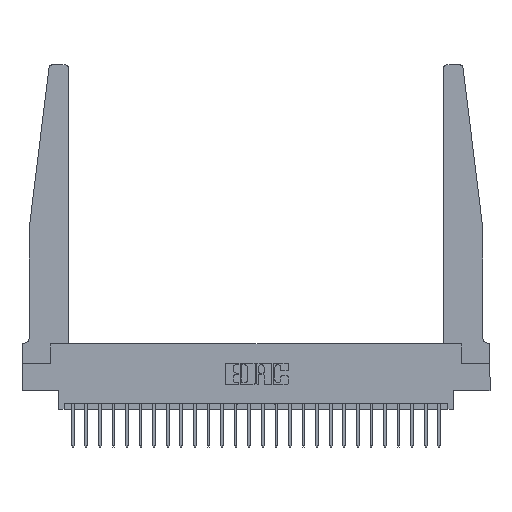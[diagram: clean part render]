
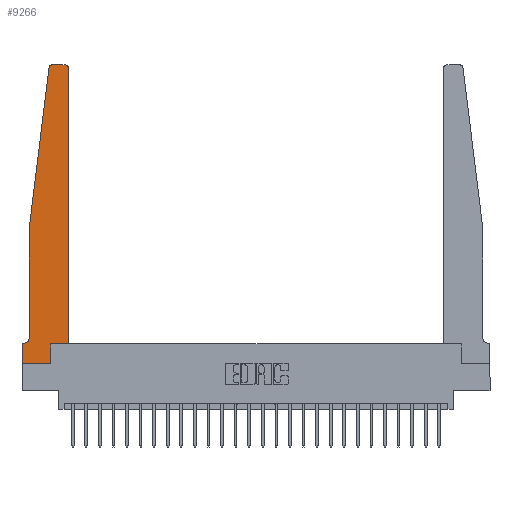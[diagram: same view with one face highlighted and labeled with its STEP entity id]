
A CAD part, top view. The second image highlights one B-rep face of the part: STEP entity #9266.
In plain terms, the highlighted planar face has unit normal (0, 0, 1).
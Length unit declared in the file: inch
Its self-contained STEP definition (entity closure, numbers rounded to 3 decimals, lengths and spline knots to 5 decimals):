
#272 = ORIENTED_EDGE ( 'NONE', *, *, #14787, .T. ) ;
#469 = EDGE_CURVE ( 'NONE', #1598, #17862, #11329, .T. ) ;
#521 = DIRECTION ( 'NONE',  ( -0.122, -0.992, 0. ) ) ;
#1453 = EDGE_CURVE ( 'NONE', #22445, #1598, #14292, .T. ) ;
#1598 = VERTEX_POINT ( 'NONE', #15333 ) ;
#2372 = CARTESIAN_POINT ( 'NONE',  ( 0.065, 0.1875, 0.37 ) ) ;
#2399 = EDGE_CURVE ( 'NONE', #22223, #10995, #5107, .T. ) ;
#2523 = EDGE_CURVE ( 'NONE', #14954, #24318, #22716, .T. ) ;
#2830 = CARTESIAN_POINT ( 'NONE',  ( 0., 0.1875, 0.37 ) ) ;
#2934 = EDGE_CURVE ( 'NONE', #22909, #4610, #3886, .T. ) ;
#3009 = CARTESIAN_POINT ( 'NONE',  ( 0.24675, 2.72367, 0.37 ) ) ;
#3243 = DIRECTION ( 'NONE',  ( 1., 0., 0. ) ) ;
#3268 = CARTESIAN_POINT ( 'NONE',  ( 0.2605, 0.18, 0.37 ) ) ;
#3551 = LINE ( 'NONE', #21809, #23583 ) ;
#3886 = LINE ( 'NONE', #2372, #8434 ) ;
#4200 = ORIENTED_EDGE ( 'NONE', *, *, #2934, .T. ) ;
#4582 = AXIS2_PLACEMENT_3D ( 'NONE', #4641, #18263, #6617 ) ;
#4610 = VERTEX_POINT ( 'NONE', #12937 ) ;
#4641 = CARTESIAN_POINT ( 'NONE',  ( 0.395, 2.72, 0.37 ) ) ;
#4689 = CARTESIAN_POINT ( 'NONE',  ( 0.425, 0.18, 0.37 ) ) ;
#4763 = ORIENTED_EDGE ( 'NONE', *, *, #2399, .T. ) ;
#4767 = EDGE_CURVE ( 'NONE', #17862, #22223, #10786, .T. ) ;
#4789 = ORIENTED_EDGE ( 'NONE', *, *, #11882, .T. ) ;
#4875 = CIRCLE ( 'NONE', #15342, 0.05 ) ;
#5107 = CIRCLE ( 'NONE', #4582, 0.03 ) ;
#5318 = CARTESIAN_POINT ( 'NONE',  ( 0.425, 0.18, 0.37 ) ) ;
#6133 = VECTOR ( 'NONE', #21604, 39.37008 ) ;
#6617 = DIRECTION ( 'NONE',  ( 1., 0., 0. ) ) ;
#6689 = EDGE_CURVE ( 'NONE', #12760, #16918, #17089, .T. ) ;
#6727 = DIRECTION ( 'NONE',  ( 1., 0., 0. ) ) ;
#6923 = CARTESIAN_POINT ( 'NONE',  ( 0.2605, 0., 0.37 ) ) ;
#7419 = CARTESIAN_POINT ( 'NONE',  ( 0.395, 2.75, 0.37 ) ) ;
#8035 = CARTESIAN_POINT ( 'NONE',  ( 0., 0., 0.37 ) ) ;
#8206 = DIRECTION ( 'NONE',  ( -1., 0., 0. ) ) ;
#8298 = CARTESIAN_POINT ( 'NONE',  ( 0.015, 0.2375, 0.37 ) ) ;
#8434 = VECTOR ( 'NONE', #8206, 39.37008 ) ;
#8600 = PLANE ( 'NONE',  #14808 ) ;
#8695 = CARTESIAN_POINT ( 'NONE',  ( 0.25, 2.75, 0.37 ) ) ;
#9102 = VECTOR ( 'NONE', #20760, 39.37008 ) ;
#9266 = ADVANCED_FACE ( 'NONE', ( #24094 ), #8600, .T. ) ;
#9939 = VECTOR ( 'NONE', #3243, 39.37008 ) ;
#10275 = DIRECTION ( 'NONE',  ( -1., 0., 0. ) ) ;
#10508 = EDGE_LOOP ( 'NONE', ( #20583, #14838, #272, #15156, #4789, #4200, #24207, #13949, #18498, #13337, #10584, #4763 ) ) ;
#10542 = EDGE_CURVE ( 'NONE', #4610, #22174, #12548, .T. ) ;
#10584 = ORIENTED_EDGE ( 'NONE', *, *, #4767, .T. ) ;
#10786 = LINE ( 'NONE', #5318, #20489 ) ;
#10872 = CARTESIAN_POINT ( 'NONE',  ( 0.27653, 2.72, 0.37 ) ) ;
#10995 = VERTEX_POINT ( 'NONE', #7419 ) ;
#11329 = LINE ( 'NONE', #13200, #17106 ) ;
#11882 = EDGE_CURVE ( 'NONE', #16918, #22909, #4875, .T. ) ;
#11920 = VECTOR ( 'NONE', #18100, 39.37008 ) ;
#12227 = CARTESIAN_POINT ( 'NONE',  ( 0.425, 2.72, 0.37 ) ) ;
#12236 = CARTESIAN_POINT ( 'NONE',  ( 0.065, 1.25, 0.37 ) ) ;
#12548 = LINE ( 'NONE', #8035, #6133 ) ;
#12760 = VERTEX_POINT ( 'NONE', #24766 ) ;
#12839 = DIRECTION ( 'NONE',  ( 1., 0., 0. ) ) ;
#12868 = CARTESIAN_POINT ( 'NONE',  ( 0., 0., 0.37 ) ) ;
#12937 = CARTESIAN_POINT ( 'NONE',  ( 0., 0.1875, 0.37 ) ) ;
#13200 = CARTESIAN_POINT ( 'NONE',  ( 0.425, 0.18, 0.37 ) ) ;
#13284 = DIRECTION ( 'NONE',  ( 1., 0., 0. ) ) ;
#13337 = ORIENTED_EDGE ( 'NONE', *, *, #469, .T. ) ;
#13538 = LINE ( 'NONE', #8695, #23221 ) ;
#13888 = CARTESIAN_POINT ( 'NONE',  ( 0.015, 0.1875, 0.37 ) ) ;
#13949 = ORIENTED_EDGE ( 'NONE', *, *, #24907, .T. ) ;
#14292 = LINE ( 'NONE', #3268, #9102 ) ;
#14787 = EDGE_CURVE ( 'NONE', #24318, #12760, #3551, .T. ) ;
#14808 = AXIS2_PLACEMENT_3D ( 'NONE', #2830, #18379, #6727 ) ;
#14838 = ORIENTED_EDGE ( 'NONE', *, *, #2523, .T. ) ;
#14954 = VERTEX_POINT ( 'NONE', #18417 ) ;
#15093 = LINE ( 'NONE', #12868, #9939 ) ;
#15156 = ORIENTED_EDGE ( 'NONE', *, *, #6689, .T. ) ;
#15333 = CARTESIAN_POINT ( 'NONE',  ( 0.2605, 0.18, 0.37 ) ) ;
#15342 = AXIS2_PLACEMENT_3D ( 'NONE', #8298, #21885, #10275 ) ;
#15537 = EDGE_CURVE ( 'NONE', #10995, #14954, #13538, .T. ) ;
#16356 = AXIS2_PLACEMENT_3D ( 'NONE', #10872, #24392, #12839 ) ;
#16918 = VERTEX_POINT ( 'NONE', #17685 ) ;
#17089 = LINE ( 'NONE', #12236, #11920 ) ;
#17106 = VECTOR ( 'NONE', #13284, 39.37008 ) ;
#17685 = CARTESIAN_POINT ( 'NONE',  ( 0.065, 0.2375, 0.37 ) ) ;
#17862 = VERTEX_POINT ( 'NONE', #4689 ) ;
#17925 = CARTESIAN_POINT ( 'NONE',  ( 0., 0., 0.37 ) ) ;
#18100 = DIRECTION ( 'NONE',  ( 0., -1., 0. ) ) ;
#18263 = DIRECTION ( 'NONE',  ( 0., 0., 1. ) ) ;
#18379 = DIRECTION ( 'NONE',  ( 0., 0., 1. ) ) ;
#18417 = CARTESIAN_POINT ( 'NONE',  ( 0.27653, 2.75, 0.37 ) ) ;
#18498 = ORIENTED_EDGE ( 'NONE', *, *, #1453, .T. ) ;
#20331 = DIRECTION ( 'NONE',  ( -1., 0., 0. ) ) ;
#20489 = VECTOR ( 'NONE', #23236, 39.37008 ) ;
#20583 = ORIENTED_EDGE ( 'NONE', *, *, #15537, .T. ) ;
#20760 = DIRECTION ( 'NONE',  ( 0., 1., 0. ) ) ;
#21604 = DIRECTION ( 'NONE',  ( 0., -1., 0. ) ) ;
#21809 = CARTESIAN_POINT ( 'NONE',  ( 0.065, 1.25, 0.37 ) ) ;
#21885 = DIRECTION ( 'NONE',  ( 0., 0., -1. ) ) ;
#22174 = VERTEX_POINT ( 'NONE', #17925 ) ;
#22223 = VERTEX_POINT ( 'NONE', #12227 ) ;
#22445 = VERTEX_POINT ( 'NONE', #6923 ) ;
#22716 = CIRCLE ( 'NONE', #16356, 0.03 ) ;
#22909 = VERTEX_POINT ( 'NONE', #13888 ) ;
#23221 = VECTOR ( 'NONE', #20331, 39.37008 ) ;
#23236 = DIRECTION ( 'NONE',  ( 0., 1., 0. ) ) ;
#23583 = VECTOR ( 'NONE', #521, 39.37008 ) ;
#24094 = FACE_OUTER_BOUND ( 'NONE', #10508, .T. ) ;
#24207 = ORIENTED_EDGE ( 'NONE', *, *, #10542, .T. ) ;
#24318 = VERTEX_POINT ( 'NONE', #3009 ) ;
#24392 = DIRECTION ( 'NONE',  ( 0., 0., 1. ) ) ;
#24766 = CARTESIAN_POINT ( 'NONE',  ( 0.065, 1.25, 0.37 ) ) ;
#24907 = EDGE_CURVE ( 'NONE', #22174, #22445, #15093, .T. ) ;
